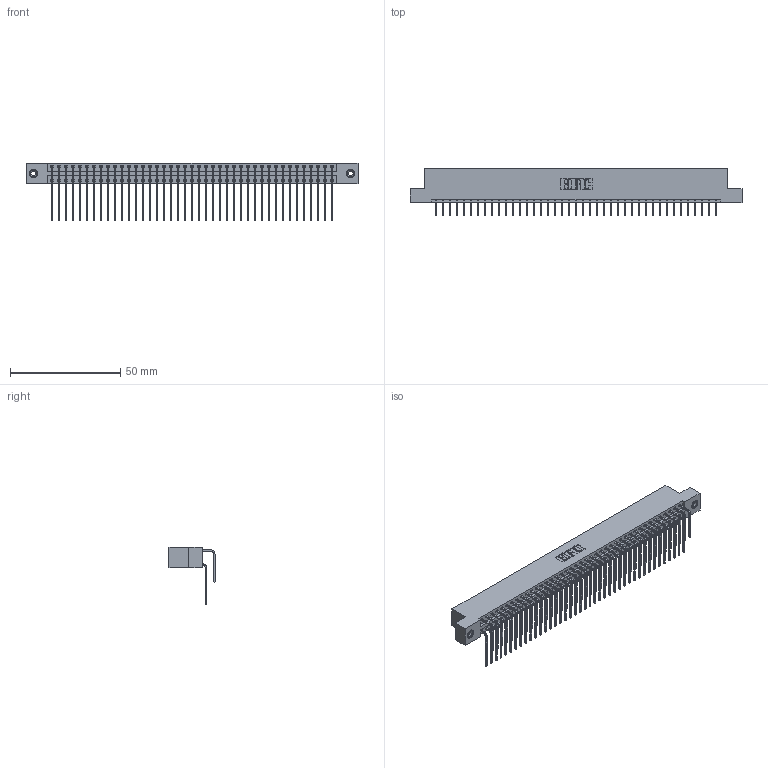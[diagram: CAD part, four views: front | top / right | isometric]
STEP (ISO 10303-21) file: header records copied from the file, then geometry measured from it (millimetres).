
FILE_DESCRIPTION (( 'STEP AP203' ), '1' );
FILE_NAME ('346-082-559-208.STEP', '2018-08-29T10:18:14', ( '' ), ( '' ), 'SwSTEP 2.0', 'SolidWorks 2016', '' );
FILE_SCHEMA (( 'CONFIG_CONTROL_DESIGN' ));
Length unit declared in the file: inch
Products named in the file (5): 345-250-001_345-250-003-102; 346-082-559-208; 346 Part_Flush Mounting Lugs - 0.156 Dia-TI; 345-292-001_558 559 Tail - 1; 345-292-001_559 Tail - 2
Assembly tree (85 placements, depth 2):
  346-082-559-208
    346 Part_Flush Mounting Lugs - 0.156 Dia-TI
    345-292-001_558 559 Tail - 1  x41
    345-292-001_559 Tail - 2  x41
    345-250-001_345-250-003-102  x2
Bounding box: 150.75 x 20.89 x 26.16 mm (x, y, z)
Volume: 15158.7 mm3; surface area: 23110.2 mm2
Topology: 85 solids, 85 shells, 4610 faces, 13667 edges, 8994 vertices
Faces by surface type: plane 3142, cylinder 1452, cone 12, torus 4
Entity records: 29862 total; most frequent: CARTESIAN_POINT 4958, ORIENTED_EDGE 4834, DIRECTION 4419, EDGE_CURVE 2417, VECTOR 2061, LINE 2061, VERTEX_POINT 1604, AXIS2_PLACEMENT_3D 1179
